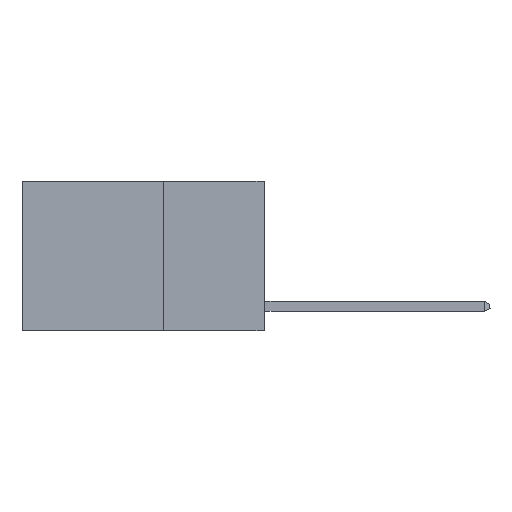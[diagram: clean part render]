
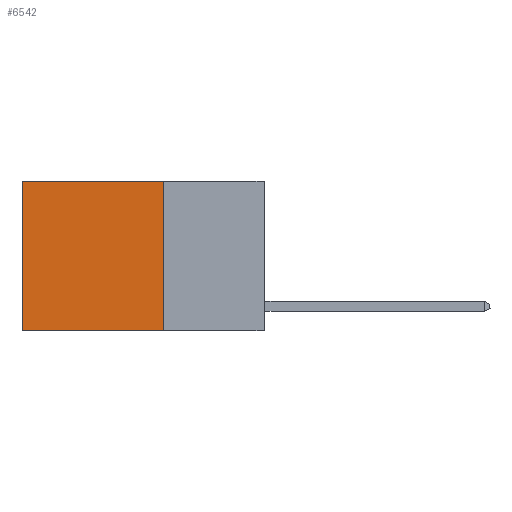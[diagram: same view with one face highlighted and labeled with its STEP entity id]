
A CAD part, left-side view. The second image highlights one B-rep face of the part: STEP entity #6542.
In plain terms, the highlighted planar face has unit normal (-1, 0, 0).
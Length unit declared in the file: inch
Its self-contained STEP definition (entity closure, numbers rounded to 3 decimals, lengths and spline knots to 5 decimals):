
#425 = CARTESIAN_POINT ( 'NONE',  ( 0.2625, 0.6, -0.37 ) ) ;
#1430 = DIRECTION ( 'NONE',  ( 0., 0., -1. ) ) ;
#1591 = EDGE_CURVE ( 'NONE', #5897, #4900, #8555, .T. ) ;
#2493 = CARTESIAN_POINT ( 'NONE',  ( 0.2625, 0.25, 0. ) ) ;
#2709 = EDGE_CURVE ( 'NONE', #11221, #8614, #12045, .T. ) ;
#2917 = DIRECTION ( 'NONE',  ( 0., 1., 0. ) ) ;
#2956 = VECTOR ( 'NONE', #10000, 39.37008 ) ;
#3130 = VECTOR ( 'NONE', #2917, 39.37008 ) ;
#3139 = DIRECTION ( 'NONE',  ( 0., 0., -1. ) ) ;
#3404 = FACE_OUTER_BOUND ( 'NONE', #4746, .T. ) ;
#3547 = PLANE ( 'NONE',  #9786 ) ;
#3945 = LINE ( 'NONE', #11228, #3130 ) ;
#4746 = EDGE_LOOP ( 'NONE', ( #9837, #8210, #10525, #12873 ) ) ;
#4900 = VERTEX_POINT ( 'NONE', #7183 ) ;
#5289 = CARTESIAN_POINT ( 'NONE',  ( 0.2625, 0.25, 0. ) ) ;
#5699 = DIRECTION ( 'NONE',  ( 1., 0., 0. ) ) ;
#5860 = CARTESIAN_POINT ( 'NONE',  ( 0.2625, 0.6, 0. ) ) ;
#5897 = VERTEX_POINT ( 'NONE', #5289 ) ;
#6542 = ADVANCED_FACE ( 'NONE', ( #3404 ), #3547, .F. ) ;
#6827 = DIRECTION ( 'NONE',  ( 0., 1., 0. ) ) ;
#7183 = CARTESIAN_POINT ( 'NONE',  ( 0.2625, 0.25, -0.37 ) ) ;
#7681 = CARTESIAN_POINT ( 'NONE',  ( 0.2625, 0.6, 0. ) ) ;
#8210 = ORIENTED_EDGE ( 'NONE', *, *, #9337, .F. ) ;
#8302 = VECTOR ( 'NONE', #3139, 39.37008 ) ;
#8555 = LINE ( 'NONE', #9499, #8302 ) ;
#8614 = VERTEX_POINT ( 'NONE', #425 ) ;
#8624 = CARTESIAN_POINT ( 'NONE',  ( 0.2625, 0.25, 0. ) ) ;
#9010 = LINE ( 'NONE', #2493, #10385 ) ;
#9337 = EDGE_CURVE ( 'NONE', #4900, #8614, #3945, .T. ) ;
#9499 = CARTESIAN_POINT ( 'NONE',  ( 0.2625, 0.25, 0. ) ) ;
#9582 = EDGE_CURVE ( 'NONE', #5897, #11221, #9010, .T. ) ;
#9786 = AXIS2_PLACEMENT_3D ( 'NONE', #8624, #5699, #1430 ) ;
#9837 = ORIENTED_EDGE ( 'NONE', *, *, #2709, .T. ) ;
#10000 = DIRECTION ( 'NONE',  ( 0., 0., -1. ) ) ;
#10385 = VECTOR ( 'NONE', #6827, 39.37008 ) ;
#10525 = ORIENTED_EDGE ( 'NONE', *, *, #1591, .F. ) ;
#11221 = VERTEX_POINT ( 'NONE', #7681 ) ;
#11228 = CARTESIAN_POINT ( 'NONE',  ( 0.2625, 0.25, -0.37 ) ) ;
#12045 = LINE ( 'NONE', #5860, #2956 ) ;
#12873 = ORIENTED_EDGE ( 'NONE', *, *, #9582, .T. ) ;
